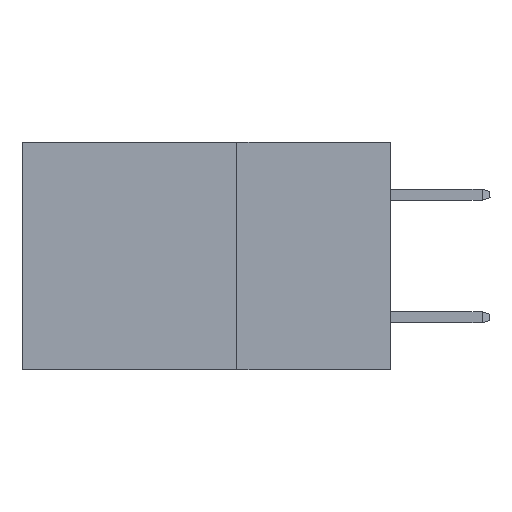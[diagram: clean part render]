
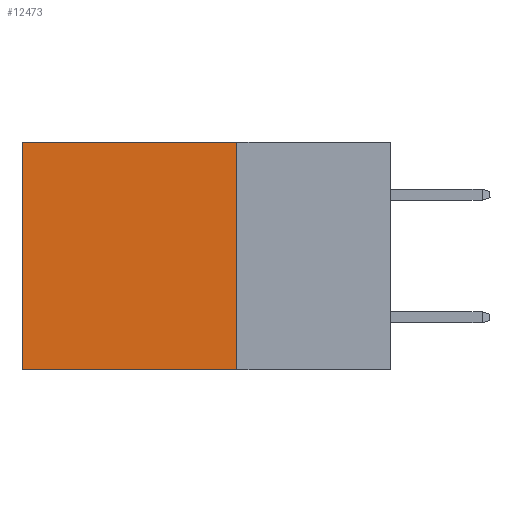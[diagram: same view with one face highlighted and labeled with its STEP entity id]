
A CAD part, left-side view. The second image highlights one B-rep face of the part: STEP entity #12473.
In plain terms, the highlighted planar face has unit normal (-1, 0, 0).
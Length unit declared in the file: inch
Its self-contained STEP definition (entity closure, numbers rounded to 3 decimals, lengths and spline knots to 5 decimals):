
#66 = ORIENTED_EDGE ( 'NONE', *, *, #11694, .T. ) ;
#74 = CARTESIAN_POINT ( 'NONE',  ( 0.2875, 0.6, 0. ) ) ;
#838 = PLANE ( 'NONE',  #2334 ) ;
#1712 = ORIENTED_EDGE ( 'NONE', *, *, #3443, .F. ) ;
#2334 = AXIS2_PLACEMENT_3D ( 'NONE', #9192, #6711, #12692 ) ;
#2570 = VECTOR ( 'NONE', #12444, 39.37008 ) ;
#3443 = EDGE_CURVE ( 'NONE', #11357, #11086, #5301, .T. ) ;
#4055 = DIRECTION ( 'NONE',  ( 0., 1., 0. ) ) ;
#4624 = VERTEX_POINT ( 'NONE', #7553 ) ;
#4700 = CARTESIAN_POINT ( 'NONE',  ( 0.2875, 0.6, 0. ) ) ;
#5164 = LINE ( 'NONE', #9974, #6623 ) ;
#5301 = LINE ( 'NONE', #11897, #15427 ) ;
#5494 = CARTESIAN_POINT ( 'NONE',  ( 0.2875, 0.25, -0.37 ) ) ;
#5680 = FACE_OUTER_BOUND ( 'NONE', #14308, .T. ) ;
#6117 = LINE ( 'NONE', #11378, #2570 ) ;
#6623 = VECTOR ( 'NONE', #4055, 39.37008 ) ;
#6711 = DIRECTION ( 'NONE',  ( 1., 0., 0. ) ) ;
#7012 = EDGE_CURVE ( 'NONE', #13131, #4624, #12333, .T. ) ;
#7553 = CARTESIAN_POINT ( 'NONE',  ( 0.2875, 0.6, -0.37 ) ) ;
#8520 = ORIENTED_EDGE ( 'NONE', *, *, #10987, .F. ) ;
#9192 = CARTESIAN_POINT ( 'NONE',  ( 0.2875, 0.25, 0. ) ) ;
#9974 = CARTESIAN_POINT ( 'NONE',  ( 0.2875, 0.25, 0. ) ) ;
#10987 = EDGE_CURVE ( 'NONE', #11086, #4624, #6117, .T. ) ;
#11086 = VERTEX_POINT ( 'NONE', #5494 ) ;
#11357 = VERTEX_POINT ( 'NONE', #14356 ) ;
#11378 = CARTESIAN_POINT ( 'NONE',  ( 0.2875, 0.25, -0.37 ) ) ;
#11694 = EDGE_CURVE ( 'NONE', #11357, #13131, #5164, .T. ) ;
#11794 = DIRECTION ( 'NONE',  ( 0., 0., -1. ) ) ;
#11897 = CARTESIAN_POINT ( 'NONE',  ( 0.2875, 0.25, 0. ) ) ;
#12092 = DIRECTION ( 'NONE',  ( 0., 0., -1. ) ) ;
#12333 = LINE ( 'NONE', #74, #15489 ) ;
#12444 = DIRECTION ( 'NONE',  ( 0., 1., 0. ) ) ;
#12473 = ADVANCED_FACE ( 'NONE', ( #5680 ), #838, .F. ) ;
#12692 = DIRECTION ( 'NONE',  ( 0., 0., -1. ) ) ;
#13131 = VERTEX_POINT ( 'NONE', #4700 ) ;
#13858 = ORIENTED_EDGE ( 'NONE', *, *, #7012, .T. ) ;
#14308 = EDGE_LOOP ( 'NONE', ( #13858, #8520, #1712, #66 ) ) ;
#14356 = CARTESIAN_POINT ( 'NONE',  ( 0.2875, 0.25, 0. ) ) ;
#15427 = VECTOR ( 'NONE', #11794, 39.37008 ) ;
#15489 = VECTOR ( 'NONE', #12092, 39.37008 ) ;
